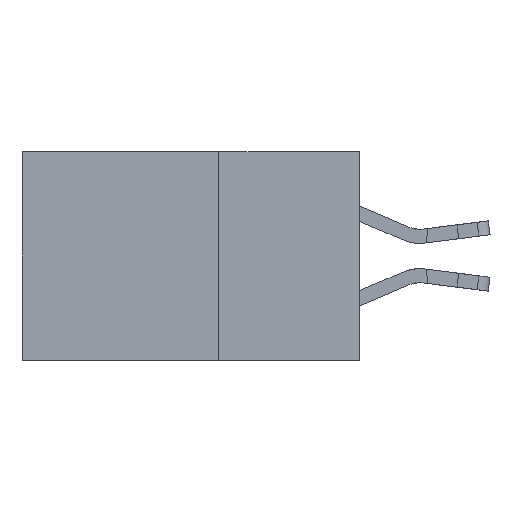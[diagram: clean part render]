
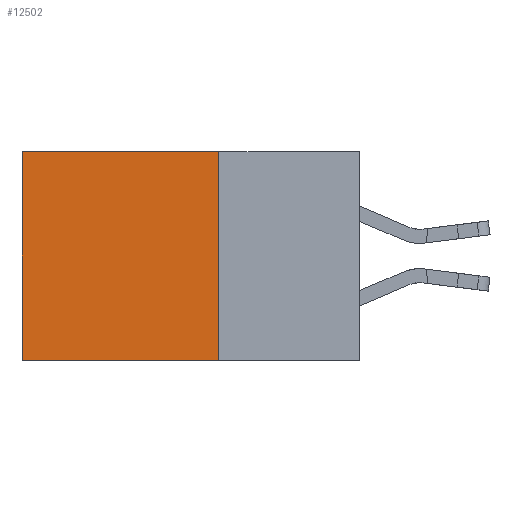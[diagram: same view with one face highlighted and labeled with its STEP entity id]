
A CAD part, left-side view. The second image highlights one B-rep face of the part: STEP entity #12502.
In plain terms, the highlighted planar face has unit normal (-1, 0, 0).
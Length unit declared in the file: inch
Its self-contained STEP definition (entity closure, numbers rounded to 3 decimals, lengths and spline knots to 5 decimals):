
#1386 = LINE ( 'NONE', #25877, #16726 ) ;
#1623 = CARTESIAN_POINT ( 'NONE',  ( 0.2875, 0.25, 0. ) ) ;
#1763 = AXIS2_PLACEMENT_3D ( 'NONE', #9702, #32326, #27260 ) ;
#3996 = VERTEX_POINT ( 'NONE', #5550 ) ;
#5520 = VERTEX_POINT ( 'NONE', #16869 ) ;
#5550 = CARTESIAN_POINT ( 'NONE',  ( 0.2875, 0.6, -0.37 ) ) ;
#6811 = CARTESIAN_POINT ( 'NONE',  ( 0.2875, 0.6, 0. ) ) ;
#7493 = EDGE_CURVE ( 'NONE', #12259, #11697, #10386, .T. ) ;
#9702 = CARTESIAN_POINT ( 'NONE',  ( 0.2875, 0.25, 0. ) ) ;
#10386 = LINE ( 'NONE', #27959, #24656 ) ;
#11045 = ORIENTED_EDGE ( 'NONE', *, *, #31323, .T. ) ;
#11697 = VERTEX_POINT ( 'NONE', #22135 ) ;
#11810 = VECTOR ( 'NONE', #16526, 39.37008 ) ;
#12115 = EDGE_CURVE ( 'NONE', #5520, #3996, #21300, .T. ) ;
#12259 = VERTEX_POINT ( 'NONE', #19814 ) ;
#12502 = ADVANCED_FACE ( 'NONE', ( #14797 ), #29708, .F. ) ;
#14797 = FACE_OUTER_BOUND ( 'NONE', #26113, .T. ) ;
#16526 = DIRECTION ( 'NONE',  ( 0., 0., -1. ) ) ;
#16726 = VECTOR ( 'NONE', #23781, 39.37008 ) ;
#16869 = CARTESIAN_POINT ( 'NONE',  ( 0.2875, 0.6, 0. ) ) ;
#17174 = ORIENTED_EDGE ( 'NONE', *, *, #7493, .F. ) ;
#18781 = LINE ( 'NONE', #1623, #26161 ) ;
#19814 = CARTESIAN_POINT ( 'NONE',  ( 0.2875, 0.25, 0. ) ) ;
#21300 = LINE ( 'NONE', #6811, #11810 ) ;
#22135 = CARTESIAN_POINT ( 'NONE',  ( 0.2875, 0.25, -0.37 ) ) ;
#23419 = ORIENTED_EDGE ( 'NONE', *, *, #12115, .T. ) ;
#23781 = DIRECTION ( 'NONE',  ( 0., 1., 0. ) ) ;
#23856 = DIRECTION ( 'NONE',  ( 0., 1., 0. ) ) ;
#24656 = VECTOR ( 'NONE', #25647, 39.37008 ) ;
#25647 = DIRECTION ( 'NONE',  ( 0., 0., -1. ) ) ;
#25877 = CARTESIAN_POINT ( 'NONE',  ( 0.2875, 0.25, -0.37 ) ) ;
#26009 = ORIENTED_EDGE ( 'NONE', *, *, #32275, .F. ) ;
#26113 = EDGE_LOOP ( 'NONE', ( #23419, #26009, #17174, #11045 ) ) ;
#26161 = VECTOR ( 'NONE', #23856, 39.37008 ) ;
#27260 = DIRECTION ( 'NONE',  ( 0., 0., -1. ) ) ;
#27959 = CARTESIAN_POINT ( 'NONE',  ( 0.2875, 0.25, 0. ) ) ;
#29708 = PLANE ( 'NONE',  #1763 ) ;
#31323 = EDGE_CURVE ( 'NONE', #12259, #5520, #18781, .T. ) ;
#32275 = EDGE_CURVE ( 'NONE', #11697, #3996, #1386, .T. ) ;
#32326 = DIRECTION ( 'NONE',  ( 1., 0., 0. ) ) ;
